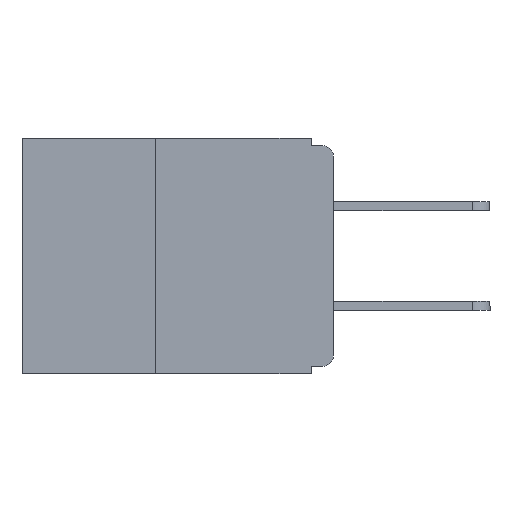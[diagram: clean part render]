
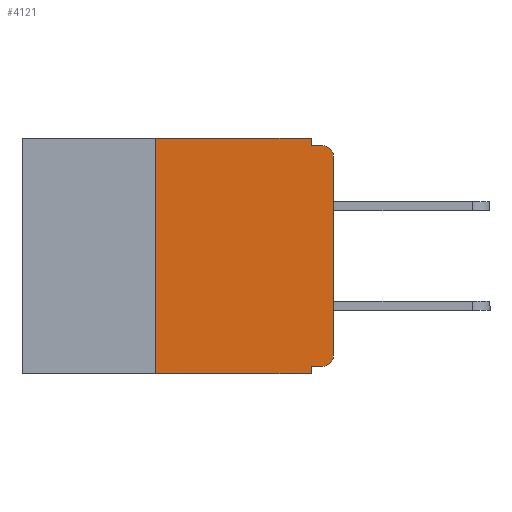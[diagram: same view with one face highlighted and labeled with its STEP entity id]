
A CAD part, left-side view. The second image highlights one B-rep face of the part: STEP entity #4121.
In plain terms, the highlighted planar face has unit normal (-1, 0, 0).
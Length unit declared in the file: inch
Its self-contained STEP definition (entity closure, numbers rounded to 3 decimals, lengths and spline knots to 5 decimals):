
#174 = PLANE ( 'NONE',  #3091 ) ;
#327 = LINE ( 'NONE', #1778, #10156 ) ;
#379 = VECTOR ( 'NONE', #2702, 39.37008 ) ;
#680 = CARTESIAN_POINT ( 'NONE',  ( 0., 0.031, 0. ) ) ;
#773 = LINE ( 'NONE', #6034, #5430 ) ;
#859 = VERTEX_POINT ( 'NONE', #23405 ) ;
#1567 = DIRECTION ( 'NONE',  ( 0., 1., 0. ) ) ;
#1778 = CARTESIAN_POINT ( 'NONE',  ( 0., 0.25, -0.33 ) ) ;
#2702 = DIRECTION ( 'NONE',  ( 0., 0., -1. ) ) ;
#3091 = AXIS2_PLACEMENT_3D ( 'NONE', #21801, #8079, #20751 ) ;
#3234 = CARTESIAN_POINT ( 'NONE',  ( 0., 0.015, -0.01 ) ) ;
#3800 = DIRECTION ( 'NONE',  ( 0., 0., 1. ) ) ;
#4121 = ADVANCED_FACE ( 'NONE', ( #5526 ), #174, .F. ) ;
#4409 = EDGE_CURVE ( 'NONE', #22037, #20791, #9769, .T. ) ;
#4432 = EDGE_CURVE ( 'NONE', #12690, #6377, #4599, .T. ) ;
#4434 = ORIENTED_EDGE ( 'NONE', *, *, #13246, .F. ) ;
#4599 = LINE ( 'NONE', #24108, #9170 ) ;
#5430 = VECTOR ( 'NONE', #5720, 39.37008 ) ;
#5519 = ORIENTED_EDGE ( 'NONE', *, *, #5915, .F. ) ;
#5526 = FACE_OUTER_BOUND ( 'NONE', #8364, .T. ) ;
#5679 = LINE ( 'NONE', #24638, #10246 ) ;
#5720 = DIRECTION ( 'NONE',  ( 0., 0., -1. ) ) ;
#5915 = EDGE_CURVE ( 'NONE', #21466, #6377, #773, .T. ) ;
#6034 = CARTESIAN_POINT ( 'NONE',  ( 0., 0.031, -0.33 ) ) ;
#6165 = CARTESIAN_POINT ( 'NONE',  ( 0., 0.031, -0.33 ) ) ;
#6307 = DIRECTION ( 'NONE',  ( 0., -1., 0. ) ) ;
#6377 = VERTEX_POINT ( 'NONE', #6165 ) ;
#6787 = CARTESIAN_POINT ( 'NONE',  ( 0., 0.437, 0. ) ) ;
#7295 = DIRECTION ( 'NONE',  ( -1., 0., 0. ) ) ;
#7720 = ORIENTED_EDGE ( 'NONE', *, *, #19563, .T. ) ;
#7816 = EDGE_CURVE ( 'NONE', #24495, #19423, #23683, .T. ) ;
#8079 = DIRECTION ( 'NONE',  ( 1., 0., 0. ) ) ;
#8316 = ORIENTED_EDGE ( 'NONE', *, *, #15879, .F. ) ;
#8364 = EDGE_LOOP ( 'NONE', ( #7720, #11358, #12005, #18417, #4434, #12173, #23538, #5519, #8316, #18647 ) ) ;
#8785 = CARTESIAN_POINT ( 'NONE',  ( 0., 0., 0. ) ) ;
#9170 = VECTOR ( 'NONE', #24076, 39.37008 ) ;
#9578 = CARTESIAN_POINT ( 'NONE',  ( 0., 0., -0.025 ) ) ;
#9769 = LINE ( 'NONE', #14639, #24399 ) ;
#10156 = VECTOR ( 'NONE', #3800, 39.37008 ) ;
#10246 = VECTOR ( 'NONE', #1567, 39.37008 ) ;
#10459 = CARTESIAN_POINT ( 'NONE',  ( 0., 0.015, -0.305 ) ) ;
#10838 = LINE ( 'NONE', #680, #379 ) ;
#11358 = ORIENTED_EDGE ( 'NONE', *, *, #17060, .T. ) ;
#11453 = CARTESIAN_POINT ( 'NONE',  ( 0., 0.25, 0. ) ) ;
#11531 = LINE ( 'NONE', #8785, #21793 ) ;
#12005 = ORIENTED_EDGE ( 'NONE', *, *, #4409, .F. ) ;
#12155 = CARTESIAN_POINT ( 'NONE',  ( 0., 0., -0.305 ) ) ;
#12173 = ORIENTED_EDGE ( 'NONE', *, *, #24020, .F. ) ;
#12405 = DIRECTION ( 'NONE',  ( 0., 0., -1. ) ) ;
#12690 = VERTEX_POINT ( 'NONE', #20292 ) ;
#12856 = VECTOR ( 'NONE', #18439, 39.37008 ) ;
#13246 = EDGE_CURVE ( 'NONE', #24555, #859, #23585, .T. ) ;
#14639 = CARTESIAN_POINT ( 'NONE',  ( 0., 0., -0.01 ) ) ;
#14763 = CARTESIAN_POINT ( 'NONE',  ( 0., 0.031, -0.01 ) ) ;
#15879 = EDGE_CURVE ( 'NONE', #24495, #21466, #5679, .T. ) ;
#16281 = EDGE_CURVE ( 'NONE', #859, #22037, #10838, .T. ) ;
#17060 = EDGE_CURVE ( 'NONE', #17169, #20791, #23909, .T. ) ;
#17169 = VERTEX_POINT ( 'NONE', #9578 ) ;
#17174 = CARTESIAN_POINT ( 'NONE',  ( 0., 0.015, -0.32 ) ) ;
#18417 = ORIENTED_EDGE ( 'NONE', *, *, #16281, .F. ) ;
#18439 = DIRECTION ( 'NONE',  ( 0., -1., 0. ) ) ;
#18647 = ORIENTED_EDGE ( 'NONE', *, *, #7816, .T. ) ;
#18944 = CARTESIAN_POINT ( 'NONE',  ( 0., 0.015, -0.025 ) ) ;
#19133 = AXIS2_PLACEMENT_3D ( 'NONE', #18944, #7295, #20855 ) ;
#19423 = VERTEX_POINT ( 'NONE', #12155 ) ;
#19563 = EDGE_CURVE ( 'NONE', #19423, #17169, #11531, .T. ) ;
#20292 = CARTESIAN_POINT ( 'NONE',  ( 0., 0.25, -0.33 ) ) ;
#20751 = DIRECTION ( 'NONE',  ( 0., 0., -1. ) ) ;
#20791 = VERTEX_POINT ( 'NONE', #3234 ) ;
#20855 = DIRECTION ( 'NONE',  ( 0., 0., -1. ) ) ;
#21466 = VERTEX_POINT ( 'NONE', #24229 ) ;
#21793 = VECTOR ( 'NONE', #22205, 39.37008 ) ;
#21801 = CARTESIAN_POINT ( 'NONE',  ( 0., 0.437, 0. ) ) ;
#22037 = VERTEX_POINT ( 'NONE', #14763 ) ;
#22205 = DIRECTION ( 'NONE',  ( 0., 0., 1. ) ) ;
#23156 = AXIS2_PLACEMENT_3D ( 'NONE', #10459, #23808, #12405 ) ;
#23405 = CARTESIAN_POINT ( 'NONE',  ( 0., 0.031, 0. ) ) ;
#23538 = ORIENTED_EDGE ( 'NONE', *, *, #4432, .T. ) ;
#23585 = LINE ( 'NONE', #6787, #12856 ) ;
#23683 = CIRCLE ( 'NONE', #23156, 0.015 ) ;
#23808 = DIRECTION ( 'NONE',  ( -1., 0., 0. ) ) ;
#23909 = CIRCLE ( 'NONE', #19133, 0.015 ) ;
#24020 = EDGE_CURVE ( 'NONE', #12690, #24555, #327, .T. ) ;
#24076 = DIRECTION ( 'NONE',  ( 0., -1., 0. ) ) ;
#24108 = CARTESIAN_POINT ( 'NONE',  ( 0., 0.437, -0.33 ) ) ;
#24229 = CARTESIAN_POINT ( 'NONE',  ( 0., 0.031, -0.32 ) ) ;
#24399 = VECTOR ( 'NONE', #6307, 39.37008 ) ;
#24495 = VERTEX_POINT ( 'NONE', #17174 ) ;
#24555 = VERTEX_POINT ( 'NONE', #11453 ) ;
#24638 = CARTESIAN_POINT ( 'NONE',  ( 0., 0., -0.32 ) ) ;
